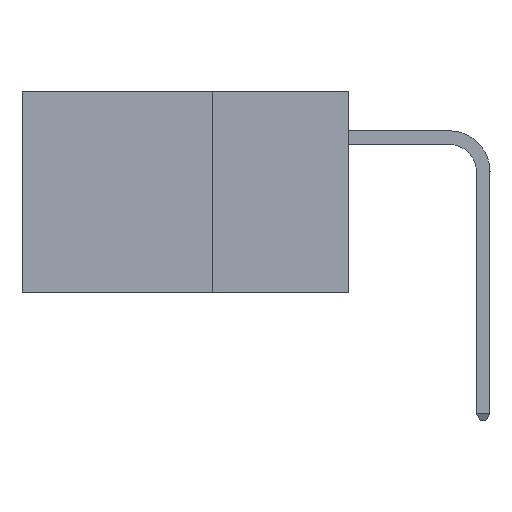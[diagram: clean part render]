
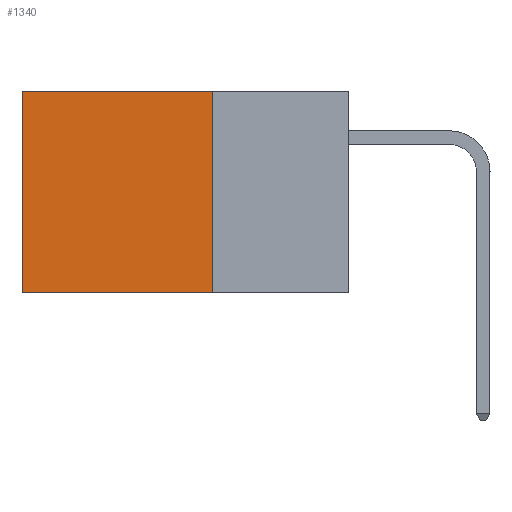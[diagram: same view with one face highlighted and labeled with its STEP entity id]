
A CAD part, left-side view. The second image highlights one B-rep face of the part: STEP entity #1340.
In plain terms, the highlighted planar face has unit normal (-1, 0, 0).
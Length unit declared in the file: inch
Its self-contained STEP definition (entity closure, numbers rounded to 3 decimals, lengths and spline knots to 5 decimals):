
#334 = CARTESIAN_POINT ( 'NONE',  ( 0.2875, 0.6, 0. ) ) ;
#484 = VECTOR ( 'NONE', #2879, 39.37008 ) ;
#667 = DIRECTION ( 'NONE',  ( 0., 0., -1. ) ) ;
#720 = DIRECTION ( 'NONE',  ( 1., 0., 0. ) ) ;
#727 = CARTESIAN_POINT ( 'NONE',  ( 0.2875, 0.25, 0. ) ) ;
#1244 = PLANE ( 'NONE',  #3643 ) ;
#1340 = ADVANCED_FACE ( 'NONE', ( #2702 ), #1244, .F. ) ;
#1512 = ORIENTED_EDGE ( 'NONE', *, *, #8234, .T. ) ;
#1699 = EDGE_CURVE ( 'NONE', #7756, #2580, #3681, .T. ) ;
#2243 = EDGE_LOOP ( 'NONE', ( #1512, #2452, #3524, #3035 ) ) ;
#2452 = ORIENTED_EDGE ( 'NONE', *, *, #1699, .F. ) ;
#2580 = VERTEX_POINT ( 'NONE', #4460 ) ;
#2702 = FACE_OUTER_BOUND ( 'NONE', #2243, .T. ) ;
#2820 = VECTOR ( 'NONE', #6305, 39.37008 ) ;
#2879 = DIRECTION ( 'NONE',  ( 0., 1., 0. ) ) ;
#3035 = ORIENTED_EDGE ( 'NONE', *, *, #4799, .T. ) ;
#3114 = CARTESIAN_POINT ( 'NONE',  ( 0.2875, 0.25, -0.37 ) ) ;
#3522 = LINE ( 'NONE', #334, #2820 ) ;
#3524 = ORIENTED_EDGE ( 'NONE', *, *, #5276, .F. ) ;
#3643 = AXIS2_PLACEMENT_3D ( 'NONE', #727, #720, #667 ) ;
#3681 = LINE ( 'NONE', #3114, #484 ) ;
#4110 = CARTESIAN_POINT ( 'NONE',  ( 0.2875, 0.25, 0. ) ) ;
#4149 = DIRECTION ( 'NONE',  ( 0., 1., 0. ) ) ;
#4460 = CARTESIAN_POINT ( 'NONE',  ( 0.2875, 0.6, -0.37 ) ) ;
#4799 = EDGE_CURVE ( 'NONE', #6888, #8443, #9690, .T. ) ;
#5276 = EDGE_CURVE ( 'NONE', #6888, #7756, #6911, .T. ) ;
#6067 = CARTESIAN_POINT ( 'NONE',  ( 0.2875, 0.25, -0.37 ) ) ;
#6305 = DIRECTION ( 'NONE',  ( 0., 0., -1. ) ) ;
#6690 = VECTOR ( 'NONE', #7150, 39.37008 ) ;
#6888 = VERTEX_POINT ( 'NONE', #8462 ) ;
#6911 = LINE ( 'NONE', #7081, #6690 ) ;
#7081 = CARTESIAN_POINT ( 'NONE',  ( 0.2875, 0.25, 0. ) ) ;
#7150 = DIRECTION ( 'NONE',  ( 0., 0., -1. ) ) ;
#7756 = VERTEX_POINT ( 'NONE', #6067 ) ;
#8000 = CARTESIAN_POINT ( 'NONE',  ( 0.2875, 0.6, 0. ) ) ;
#8234 = EDGE_CURVE ( 'NONE', #8443, #2580, #3522, .T. ) ;
#8443 = VERTEX_POINT ( 'NONE', #8000 ) ;
#8462 = CARTESIAN_POINT ( 'NONE',  ( 0.2875, 0.25, 0. ) ) ;
#9590 = VECTOR ( 'NONE', #4149, 39.37008 ) ;
#9690 = LINE ( 'NONE', #4110, #9590 ) ;
